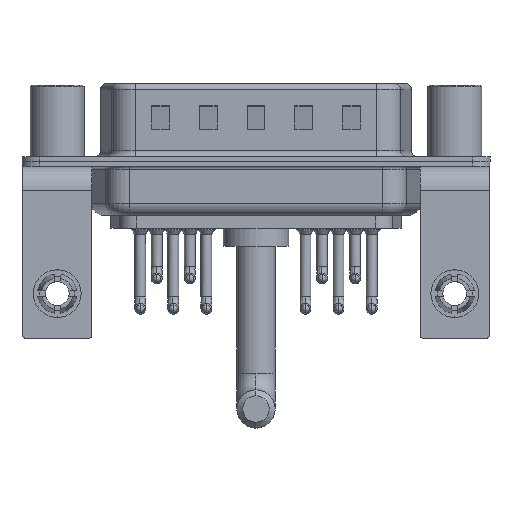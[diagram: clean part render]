
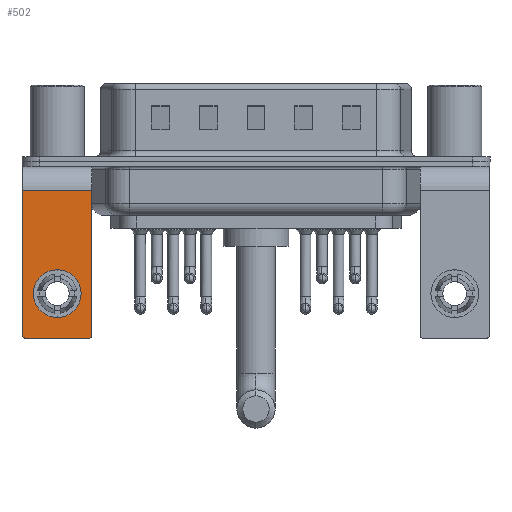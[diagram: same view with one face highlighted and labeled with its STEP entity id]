
A CAD part, front view. The second image highlights one B-rep face of the part: STEP entity #502.
In plain terms, the highlighted planar face has unit normal (0, -1, 0).
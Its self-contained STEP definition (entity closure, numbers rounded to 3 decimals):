
#502 = ADVANCED_FACE ( 'NONE', ( #22974, #14544 ), #16287, .F. ) ;
#913 = VERTEX_POINT ( 'NONE', #3922 ) ;
#1464 = CARTESIAN_POINT ( 'NONE',  ( 0., -6.25, -13.07 ) ) ;
#1591 = CIRCLE ( 'NONE', #9723, 2. ) ;
#1915 = DIRECTION ( 'NONE',  ( -1., 0., 0. ) ) ;
#2331 = LINE ( 'NONE', #6222, #11190 ) ;
#2526 = CIRCLE ( 'NONE', #17510, 0.25 ) ;
#2565 = CARTESIAN_POINT ( 'NONE',  ( -2.9, -6.25, -2.4 ) ) ;
#2888 = VECTOR ( 'NONE', #24669, 1000. ) ;
#2993 = EDGE_CURVE ( 'NONE', #13890, #18930, #1591, .T. ) ;
#3671 = LINE ( 'NONE', #21900, #8093 ) ;
#3723 = ORIENTED_EDGE ( 'NONE', *, *, #11197, .F. ) ;
#3922 = CARTESIAN_POINT ( 'NONE',  ( 2.65, -6.25, -14.8 ) ) ;
#4022 = CARTESIAN_POINT ( 'NONE',  ( 2.9, -6.25, -14.55 ) ) ;
#4092 = EDGE_CURVE ( 'NONE', #913, #18102, #2526, .T. ) ;
#4167 = CARTESIAN_POINT ( 'NONE',  ( 0., -6.25, -11.07 ) ) ;
#4281 = VERTEX_POINT ( 'NONE', #15532 ) ;
#4528 = DIRECTION ( 'NONE',  ( 0., -1., 0. ) ) ;
#4571 = DIRECTION ( 'NONE',  ( 0., 0., -1. ) ) ;
#4613 = DIRECTION ( 'NONE',  ( 0., 1., 0. ) ) ;
#5304 = VERTEX_POINT ( 'NONE', #23252 ) ;
#5352 = EDGE_CURVE ( 'NONE', #913, #7324, #3671, .T. ) ;
#5542 = AXIS2_PLACEMENT_3D ( 'NONE', #8273, #4528, #21019 ) ;
#6077 = EDGE_LOOP ( 'NONE', ( #22201, #7918, #24078, #20132, #3723, #11163 ) ) ;
#6088 = DIRECTION ( 'NONE',  ( 0., 0., 1. ) ) ;
#6222 = CARTESIAN_POINT ( 'NONE',  ( 2.9, -6.25, -2.4 ) ) ;
#7324 = VERTEX_POINT ( 'NONE', #24646 ) ;
#7396 = EDGE_CURVE ( 'NONE', #4281, #7324, #13699, .T. ) ;
#7739 = VECTOR ( 'NONE', #4571, 1000. ) ;
#7871 = CIRCLE ( 'NONE', #14320, 2. ) ;
#7918 = ORIENTED_EDGE ( 'NONE', *, *, #7396, .T. ) ;
#8093 = VECTOR ( 'NONE', #1915, 1000. ) ;
#8273 = CARTESIAN_POINT ( 'NONE',  ( -2.65, -6.25, -14.55 ) ) ;
#9723 = AXIS2_PLACEMENT_3D ( 'NONE', #4167, #14489, #12334 ) ;
#10051 = CARTESIAN_POINT ( 'NONE',  ( 2.65, -6.25, -14.55 ) ) ;
#10231 = CARTESIAN_POINT ( 'NONE',  ( 0., -6.25, -9.07 ) ) ;
#11163 = ORIENTED_EDGE ( 'NONE', *, *, #21477, .T. ) ;
#11190 = VECTOR ( 'NONE', #22719, 1000. ) ;
#11197 = EDGE_CURVE ( 'NONE', #20097, #18102, #22791, .T. ) ;
#12331 = ORIENTED_EDGE ( 'NONE', *, *, #23972, .T. ) ;
#12334 = DIRECTION ( 'NONE',  ( 0., 0., 1. ) ) ;
#13416 = AXIS2_PLACEMENT_3D ( 'NONE', #20847, #4613, #6088 ) ;
#13699 = CIRCLE ( 'NONE', #5542, 0.25 ) ;
#13890 = VERTEX_POINT ( 'NONE', #10231 ) ;
#14206 = CARTESIAN_POINT ( 'NONE',  ( 2.9, -6.25, -2.4 ) ) ;
#14320 = AXIS2_PLACEMENT_3D ( 'NONE', #24793, #16883, #22903 ) ;
#14489 = DIRECTION ( 'NONE',  ( 0., 1., 0. ) ) ;
#14544 = FACE_OUTER_BOUND ( 'NONE', #6077, .T. ) ;
#15532 = CARTESIAN_POINT ( 'NONE',  ( -2.9, -6.25, -14.55 ) ) ;
#16287 = PLANE ( 'NONE',  #13416 ) ;
#16809 = CARTESIAN_POINT ( 'NONE',  ( 2.9, -6.25, -2.4 ) ) ;
#16883 = DIRECTION ( 'NONE',  ( 0., 1., 0. ) ) ;
#17510 = AXIS2_PLACEMENT_3D ( 'NONE', #10051, #22257, #22528 ) ;
#17890 = EDGE_LOOP ( 'NONE', ( #12331, #21857 ) ) ;
#18102 = VERTEX_POINT ( 'NONE', #4022 ) ;
#18930 = VERTEX_POINT ( 'NONE', #1464 ) ;
#20097 = VERTEX_POINT ( 'NONE', #16809 ) ;
#20132 = ORIENTED_EDGE ( 'NONE', *, *, #4092, .T. ) ;
#20667 = EDGE_CURVE ( 'NONE', #5304, #4281, #22936, .T. ) ;
#20847 = CARTESIAN_POINT ( 'NONE',  ( 2.9, -6.25, -2.4 ) ) ;
#21019 = DIRECTION ( 'NONE',  ( 0., 0., 1. ) ) ;
#21477 = EDGE_CURVE ( 'NONE', #20097, #5304, #2331, .T. ) ;
#21857 = ORIENTED_EDGE ( 'NONE', *, *, #2993, .T. ) ;
#21900 = CARTESIAN_POINT ( 'NONE',  ( 2.9, -6.25, -14.8 ) ) ;
#22201 = ORIENTED_EDGE ( 'NONE', *, *, #20667, .T. ) ;
#22257 = DIRECTION ( 'NONE',  ( 0., -1., 0. ) ) ;
#22528 = DIRECTION ( 'NONE',  ( 0., 0., 1. ) ) ;
#22719 = DIRECTION ( 'NONE',  ( -1., 0., 0. ) ) ;
#22791 = LINE ( 'NONE', #14206, #2888 ) ;
#22903 = DIRECTION ( 'NONE',  ( 0., 0., 1. ) ) ;
#22936 = LINE ( 'NONE', #2565, #7739 ) ;
#22974 = FACE_BOUND ( 'NONE', #17890, .T. ) ;
#23252 = CARTESIAN_POINT ( 'NONE',  ( -2.9, -6.25, -2.4 ) ) ;
#23972 = EDGE_CURVE ( 'NONE', #18930, #13890, #7871, .T. ) ;
#24078 = ORIENTED_EDGE ( 'NONE', *, *, #5352, .F. ) ;
#24646 = CARTESIAN_POINT ( 'NONE',  ( -2.65, -6.25, -14.8 ) ) ;
#24669 = DIRECTION ( 'NONE',  ( 0., 0., -1. ) ) ;
#24793 = CARTESIAN_POINT ( 'NONE',  ( 0., -6.25, -11.07 ) ) ;
